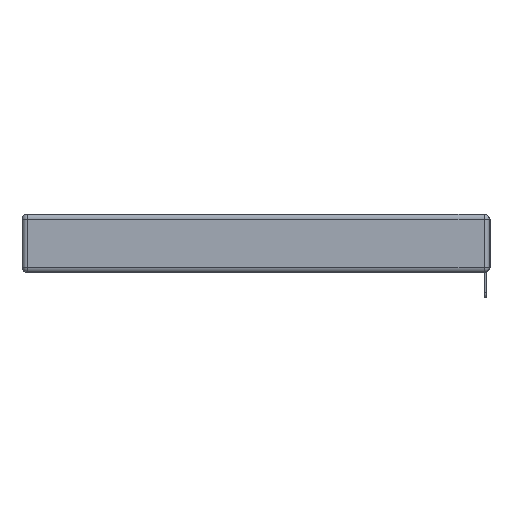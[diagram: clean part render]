
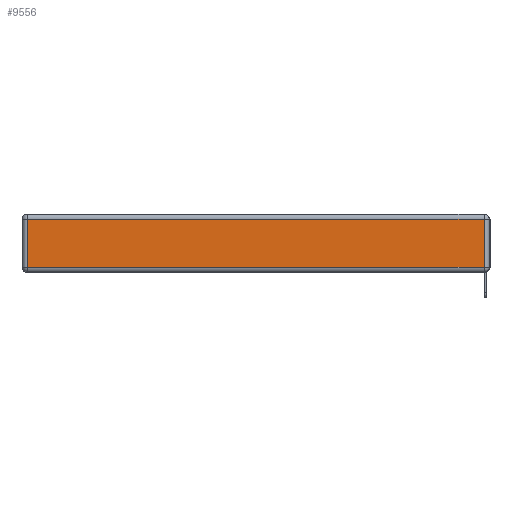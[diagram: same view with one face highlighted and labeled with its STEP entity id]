
A CAD part, left-side view. The second image highlights one B-rep face of the part: STEP entity #9556.
In plain terms, the highlighted planar face has unit normal (-1, 0, 0).
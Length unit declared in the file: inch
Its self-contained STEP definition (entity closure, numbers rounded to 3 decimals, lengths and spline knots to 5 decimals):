
#1282 = PLANE ( 'NONE',  #10083 ) ;
#1917 = CARTESIAN_POINT ( 'NONE',  ( 0., 0.03, -0.343 ) ) ;
#2038 = EDGE_LOOP ( 'NONE', ( #17346, #8506, #2758, #17376 ) ) ;
#2758 = ORIENTED_EDGE ( 'NONE', *, *, #9995, .T. ) ;
#3119 = VECTOR ( 'NONE', #15734, 39.37008 ) ;
#3809 = VERTEX_POINT ( 'NONE', #13552 ) ;
#4224 = LINE ( 'NONE', #16138, #8460 ) ;
#4658 = CARTESIAN_POINT ( 'NONE',  ( 0., 0., -0.313 ) ) ;
#4931 = CARTESIAN_POINT ( 'NONE',  ( 0., 2.72, -0.313 ) ) ;
#5193 = EDGE_CURVE ( 'NONE', #13840, #5367, #12749, .T. ) ;
#5367 = VERTEX_POINT ( 'NONE', #13453 ) ;
#7319 = LINE ( 'NONE', #12783, #3119 ) ;
#7784 = VECTOR ( 'NONE', #9802, 39.37008 ) ;
#8460 = VECTOR ( 'NONE', #10926, 39.37008 ) ;
#8506 = ORIENTED_EDGE ( 'NONE', *, *, #5193, .T. ) ;
#9556 = ADVANCED_FACE ( 'NONE', ( #9705 ), #1282, .T. ) ;
#9705 = FACE_OUTER_BOUND ( 'NONE', #2038, .T. ) ;
#9802 = DIRECTION ( 'NONE',  ( 0., 0., 1. ) ) ;
#9995 = EDGE_CURVE ( 'NONE', #5367, #3809, #4224, .T. ) ;
#10083 = AXIS2_PLACEMENT_3D ( 'NONE', #15083, #11128, #13642 ) ;
#10926 = DIRECTION ( 'NONE',  ( 0., 1., 0. ) ) ;
#11006 = VERTEX_POINT ( 'NONE', #4931 ) ;
#11128 = DIRECTION ( 'NONE',  ( -1., 0., 0. ) ) ;
#12749 = LINE ( 'NONE', #1917, #7784 ) ;
#12783 = CARTESIAN_POINT ( 'NONE',  ( 0., 2.72, -0.343 ) ) ;
#12973 = CARTESIAN_POINT ( 'NONE',  ( 0., 0.03, -0.313 ) ) ;
#13307 = VECTOR ( 'NONE', #15576, 39.37008 ) ;
#13453 = CARTESIAN_POINT ( 'NONE',  ( 0., 0.03, -0.03 ) ) ;
#13552 = CARTESIAN_POINT ( 'NONE',  ( 0., 2.72, -0.03 ) ) ;
#13642 = DIRECTION ( 'NONE',  ( 0., 0., 1. ) ) ;
#13840 = VERTEX_POINT ( 'NONE', #12973 ) ;
#15083 = CARTESIAN_POINT ( 'NONE',  ( 0., 0., -0.343 ) ) ;
#15370 = EDGE_CURVE ( 'NONE', #11006, #13840, #16927, .T. ) ;
#15576 = DIRECTION ( 'NONE',  ( 0., -1., 0. ) ) ;
#15734 = DIRECTION ( 'NONE',  ( 0., 0., -1. ) ) ;
#15763 = EDGE_CURVE ( 'NONE', #3809, #11006, #7319, .T. ) ;
#16138 = CARTESIAN_POINT ( 'NONE',  ( 0., 2.75, -0.03 ) ) ;
#16927 = LINE ( 'NONE', #4658, #13307 ) ;
#17346 = ORIENTED_EDGE ( 'NONE', *, *, #15370, .T. ) ;
#17376 = ORIENTED_EDGE ( 'NONE', *, *, #15763, .T. ) ;
